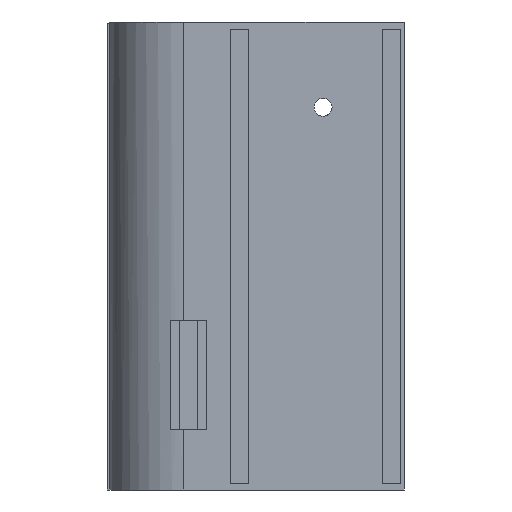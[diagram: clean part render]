
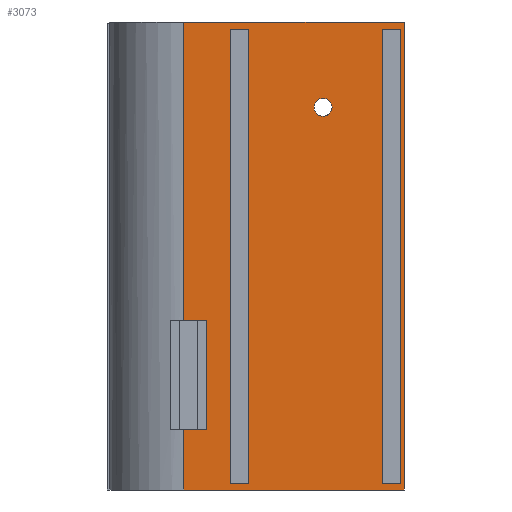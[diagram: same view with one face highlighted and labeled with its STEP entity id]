
A CAD part, left-side view. The second image highlights one B-rep face of the part: STEP entity #3073.
In plain terms, the highlighted planar face has unit normal (-1, 0, 0).
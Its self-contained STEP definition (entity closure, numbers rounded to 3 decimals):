
#45 = DIRECTION ( 'NONE',  ( 1., 0., 0. ) ) ;
#64 = PLANE ( 'NONE',  #1940 ) ;
#72 = LINE ( 'NONE', #2328, #3206 ) ;
#111 = VECTOR ( 'NONE', #2991, 1000. ) ;
#130 = VERTEX_POINT ( 'NONE', #3836 ) ;
#256 = CARTESIAN_POINT ( 'NONE',  ( -13., 25.767, 27. ) ) ;
#277 = EDGE_CURVE ( 'NONE', #809, #130, #2554, .T. ) ;
#279 = VERTEX_POINT ( 'NONE', #766 ) ;
#306 = VECTOR ( 'NONE', #3959, 1000. ) ;
#309 = VECTOR ( 'NONE', #4447, 1000. ) ;
#541 = VECTOR ( 'NONE', #4856, 1000. ) ;
#565 = CARTESIAN_POINT ( 'NONE',  ( -13., 27.9, 27. ) ) ;
#600 = LINE ( 'NONE', #3277, #5051 ) ;
#694 = LINE ( 'NONE', #3696, #4126 ) ;
#716 = DIRECTION ( 'NONE',  ( 0., 1., 0. ) ) ;
#735 = VERTEX_POINT ( 'NONE', #1529 ) ;
#753 = VECTOR ( 'NONE', #3165, 1000. ) ;
#766 = CARTESIAN_POINT ( 'NONE',  ( -13., 18., 0. ) ) ;
#776 = CARTESIAN_POINT ( 'NONE',  ( -13., 18., 75. ) ) ;
#788 = FACE_BOUND ( 'NONE', #4146, .T. ) ;
#809 = VERTEX_POINT ( 'NONE', #967 ) ;
#812 = EDGE_CURVE ( 'NONE', #2594, #1449, #3442, .T. ) ;
#868 = VECTOR ( 'NONE', #1531, 1000. ) ;
#870 = ORIENTED_EDGE ( 'NONE', *, *, #277, .T. ) ;
#967 = CARTESIAN_POINT ( 'NONE',  ( -13., 21.9, 9. ) ) ;
#1011 = DIRECTION ( 'NONE',  ( 0., 1., 0. ) ) ;
#1033 = VERTEX_POINT ( 'NONE', #3607 ) ;
#1078 = LINE ( 'NONE', #1996, #753 ) ;
#1093 = EDGE_CURVE ( 'NONE', #1449, #4776, #1078, .T. ) ;
#1142 = DIRECTION ( 'NONE',  ( 0., 0., -1. ) ) ;
#1184 = EDGE_CURVE ( 'NONE', #1410, #2594, #4194, .T. ) ;
#1189 = LINE ( 'NONE', #1714, #2978 ) ;
#1203 = ORIENTED_EDGE ( 'NONE', *, *, #1184, .T. ) ;
#1209 = CARTESIAN_POINT ( 'NONE',  ( -13., 45.608, -1. ) ) ;
#1211 = EDGE_CURVE ( 'NONE', #279, #2295, #694, .T. ) ;
#1246 = DIRECTION ( 'NONE',  ( 0., 0., 1. ) ) ;
#1258 = DIRECTION ( 'NONE',  ( 0., -1., 0. ) ) ;
#1300 = VECTOR ( 'NONE', #2742, 1000. ) ;
#1305 = VECTOR ( 'NONE', #1142, 1000. ) ;
#1398 = AXIS2_PLACEMENT_3D ( 'NONE', #2702, #1466, #716 ) ;
#1407 = CARTESIAN_POINT ( 'NONE',  ( -13., -10., 75. ) ) ;
#1410 = VERTEX_POINT ( 'NONE', #3019 ) ;
#1449 = VERTEX_POINT ( 'NONE', #2190 ) ;
#1466 = DIRECTION ( 'NONE',  ( 1., 0., 0. ) ) ;
#1473 = CARTESIAN_POINT ( 'NONE',  ( -13., 15., 0. ) ) ;
#1498 = EDGE_CURVE ( 'NONE', #2847, #5213, #3620, .T. ) ;
#1529 = CARTESIAN_POINT ( 'NONE',  ( -13., 4.241, 62.126 ) ) ;
#1531 = DIRECTION ( 'NONE',  ( 0., 0., 1. ) ) ;
#1541 = CARTESIAN_POINT ( 'NONE',  ( -13., -10.668, -1. ) ) ;
#1561 = ORIENTED_EDGE ( 'NONE', *, *, #812, .T. ) ;
#1586 = VERTEX_POINT ( 'NONE', #3245 ) ;
#1656 = EDGE_LOOP ( 'NONE', ( #5105, #1727, #4895, #870, #1885, #2626, #4781, #1888 ) ) ;
#1658 = EDGE_CURVE ( 'NONE', #2889, #1033, #1189, .T. ) ;
#1691 = ORIENTED_EDGE ( 'NONE', *, *, #2032, .T. ) ;
#1714 = CARTESIAN_POINT ( 'NONE',  ( -13., 15., 75. ) ) ;
#1727 = ORIENTED_EDGE ( 'NONE', *, *, #1498, .T. ) ;
#1779 = VERTEX_POINT ( 'NONE', #3833 ) ;
#1885 = ORIENTED_EDGE ( 'NONE', *, *, #2481, .F. ) ;
#1888 = ORIENTED_EDGE ( 'NONE', *, *, #3586, .T. ) ;
#1911 = ORIENTED_EDGE ( 'NONE', *, *, #3140, .T. ) ;
#1933 = CARTESIAN_POINT ( 'NONE',  ( -13., -7., 0. ) ) ;
#1940 = AXIS2_PLACEMENT_3D ( 'NONE', #4888, #45, #4908 ) ;
#1996 = CARTESIAN_POINT ( 'NONE',  ( -13., -10., 0. ) ) ;
#2032 = EDGE_CURVE ( 'NONE', #4776, #1410, #4238, .T. ) ;
#2061 = EDGE_CURVE ( 'NONE', #1779, #2847, #3991, .T. ) ;
#2190 = CARTESIAN_POINT ( 'NONE',  ( -13., -10., 0. ) ) ;
#2243 = EDGE_CURVE ( 'NONE', #1033, #279, #3732, .T. ) ;
#2295 = VERTEX_POINT ( 'NONE', #776 ) ;
#2301 = ORIENTED_EDGE ( 'NONE', *, *, #1211, .T. ) ;
#2314 = ORIENTED_EDGE ( 'NONE', *, *, #2830, .T. ) ;
#2328 = CARTESIAN_POINT ( 'NONE',  ( -13., 15.471, 76.189 ) ) ;
#2381 = FACE_BOUND ( 'NONE', #3193, .T. ) ;
#2424 = DIRECTION ( 'NONE',  ( 0., -1., 0. ) ) ;
#2453 = DIRECTION ( 'NONE',  ( 0., 0., -1. ) ) ;
#2481 = EDGE_CURVE ( 'NONE', #2687, #130, #2963, .T. ) ;
#2554 = LINE ( 'NONE', #3480, #3827 ) ;
#2555 = ORIENTED_EDGE ( 'NONE', *, *, #1658, .T. ) ;
#2594 = VERTEX_POINT ( 'NONE', #2985 ) ;
#2626 = ORIENTED_EDGE ( 'NONE', *, *, #2967, .T. ) ;
#2687 = VERTEX_POINT ( 'NONE', #3090 ) ;
#2700 = VECTOR ( 'NONE', #2453, 1000. ) ;
#2702 = CARTESIAN_POINT ( 'NONE',  ( -13., 2.757, 62.126 ) ) ;
#2712 = CARTESIAN_POINT ( 'NONE',  ( -13., 21.9, 27. ) ) ;
#2742 = DIRECTION ( 'NONE',  ( 0., 1., 0. ) ) ;
#2830 = EDGE_CURVE ( 'NONE', #735, #735, #3346, .T. ) ;
#2847 = VERTEX_POINT ( 'NONE', #256 ) ;
#2889 = VERTEX_POINT ( 'NONE', #4766 ) ;
#2957 = FACE_OUTER_BOUND ( 'NONE', #1656, .T. ) ;
#2963 = LINE ( 'NONE', #4116, #541 ) ;
#2967 = EDGE_CURVE ( 'NONE', #2687, #4137, #3274, .T. ) ;
#2978 = VECTOR ( 'NONE', #4921, 1000. ) ;
#2985 = CARTESIAN_POINT ( 'NONE',  ( -13., -10., 75. ) ) ;
#2991 = DIRECTION ( 'NONE',  ( 0., 0., -1. ) ) ;
#3019 = CARTESIAN_POINT ( 'NONE',  ( -13., -7., 75. ) ) ;
#3073 = ADVANCED_FACE ( 'NONE', ( #2381, #2957, #788, #4988 ), #64, .F. ) ;
#3077 = VECTOR ( 'NONE', #3572, 1000. ) ;
#3090 = CARTESIAN_POINT ( 'NONE',  ( -13., 25.767, -1. ) ) ;
#3097 = EDGE_LOOP ( 'NONE', ( #2314 ) ) ;
#3140 = EDGE_CURVE ( 'NONE', #2295, #2889, #600, .T. ) ;
#3165 = DIRECTION ( 'NONE',  ( 0., 1., 0. ) ) ;
#3171 = CARTESIAN_POINT ( 'NONE',  ( -13., 25.767, -1. ) ) ;
#3172 = DIRECTION ( 'NONE',  ( 0., 1., 0. ) ) ;
#3183 = CARTESIAN_POINT ( 'NONE',  ( -13., -10.668, -1. ) ) ;
#3193 = EDGE_LOOP ( 'NONE', ( #1911, #2555, #4810, #2301 ) ) ;
#3206 = VECTOR ( 'NONE', #3172, 1000. ) ;
#3245 = CARTESIAN_POINT ( 'NONE',  ( -13., -10.668, 76.189 ) ) ;
#3274 = LINE ( 'NONE', #1209, #4664 ) ;
#3277 = CARTESIAN_POINT ( 'NONE',  ( -13., 18., 75. ) ) ;
#3346 = CIRCLE ( 'NONE', #1398, 1.484 ) ;
#3398 = LINE ( 'NONE', #1541, #3077 ) ;
#3442 = LINE ( 'NONE', #1407, #111 ) ;
#3480 = CARTESIAN_POINT ( 'NONE',  ( -13., 21.9, 9. ) ) ;
#3572 = DIRECTION ( 'NONE',  ( 0., 0., 1. ) ) ;
#3586 = EDGE_CURVE ( 'NONE', #1586, #1779, #72, .T. ) ;
#3607 = CARTESIAN_POINT ( 'NONE',  ( -13., 15., 0. ) ) ;
#3620 = LINE ( 'NONE', #565, #306 ) ;
#3693 = EDGE_CURVE ( 'NONE', #5213, #809, #3966, .T. ) ;
#3696 = CARTESIAN_POINT ( 'NONE',  ( -13., 18., 0. ) ) ;
#3732 = LINE ( 'NONE', #1473, #1300 ) ;
#3827 = VECTOR ( 'NONE', #1011, 1000. ) ;
#3833 = CARTESIAN_POINT ( 'NONE',  ( -13., 25.767, 76.189 ) ) ;
#3836 = CARTESIAN_POINT ( 'NONE',  ( -13., 25.767, 9. ) ) ;
#3959 = DIRECTION ( 'NONE',  ( 0., -1., 0. ) ) ;
#3966 = LINE ( 'NONE', #4882, #2700 ) ;
#3991 = LINE ( 'NONE', #3171, #1305 ) ;
#4060 = EDGE_CURVE ( 'NONE', #4137, #1586, #3398, .T. ) ;
#4116 = CARTESIAN_POINT ( 'NONE',  ( -13., 25.767, -1. ) ) ;
#4126 = VECTOR ( 'NONE', #1246, 1000. ) ;
#4137 = VERTEX_POINT ( 'NONE', #3183 ) ;
#4146 = EDGE_LOOP ( 'NONE', ( #1691, #1203, #1561, #4732 ) ) ;
#4194 = LINE ( 'NONE', #5281, #309 ) ;
#4238 = LINE ( 'NONE', #1933, #868 ) ;
#4447 = DIRECTION ( 'NONE',  ( 0., -1., 0. ) ) ;
#4632 = CARTESIAN_POINT ( 'NONE',  ( -13., -7., 0. ) ) ;
#4664 = VECTOR ( 'NONE', #2424, 1000. ) ;
#4732 = ORIENTED_EDGE ( 'NONE', *, *, #1093, .T. ) ;
#4766 = CARTESIAN_POINT ( 'NONE',  ( -13., 15., 75. ) ) ;
#4776 = VERTEX_POINT ( 'NONE', #4632 ) ;
#4781 = ORIENTED_EDGE ( 'NONE', *, *, #4060, .T. ) ;
#4810 = ORIENTED_EDGE ( 'NONE', *, *, #2243, .T. ) ;
#4856 = DIRECTION ( 'NONE',  ( 0., 0., 1. ) ) ;
#4882 = CARTESIAN_POINT ( 'NONE',  ( -13., 21.9, 27. ) ) ;
#4888 = CARTESIAN_POINT ( 'NONE',  ( -13., 39.89, -1. ) ) ;
#4895 = ORIENTED_EDGE ( 'NONE', *, *, #3693, .T. ) ;
#4908 = DIRECTION ( 'NONE',  ( 0., -1., 0. ) ) ;
#4921 = DIRECTION ( 'NONE',  ( 0., 0., -1. ) ) ;
#4988 = FACE_BOUND ( 'NONE', #3097, .T. ) ;
#5051 = VECTOR ( 'NONE', #1258, 1000. ) ;
#5105 = ORIENTED_EDGE ( 'NONE', *, *, #2061, .T. ) ;
#5213 = VERTEX_POINT ( 'NONE', #2712 ) ;
#5281 = CARTESIAN_POINT ( 'NONE',  ( -13., -7., 75. ) ) ;
